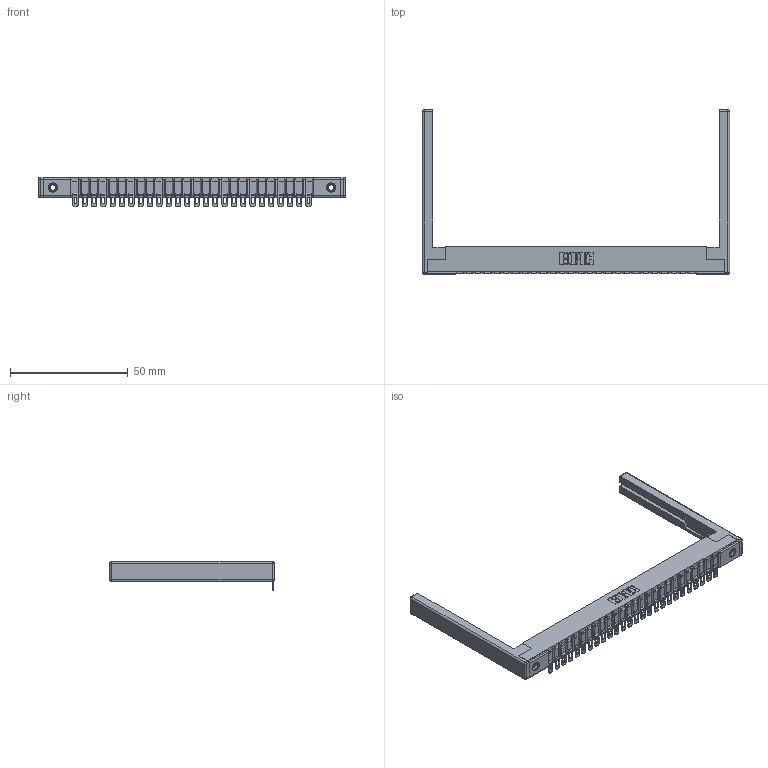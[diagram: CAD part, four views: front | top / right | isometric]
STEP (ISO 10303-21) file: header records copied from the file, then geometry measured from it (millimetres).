
FILE_DESCRIPTION (( 'STEP AP203' ), '1' );
FILE_NAME ('307-026-554-168.STEP', '2019-09-05T02:14:57', ( '' ), ( '' ), 'SwSTEP 2.0', 'SolidWorks 2016', '' );
FILE_SCHEMA (( 'CONFIG_CONTROL_DESIGN' ));
Length unit declared in the file: inch
Products named in the file (5): 307-026-554-168; 307 Part_.156 Dia Mounting Holes; 307-220-068; 345-250-001_345-250-001-102; 307-290-002_554
Assembly tree (31 placements, depth 2):
  307-026-554-168
    307 Part_.156 Dia Mounting Holes
    307-290-002_554  x26
    307-220-068  x2
    345-250-001_345-250-001-102  x2
Bounding box: 130.45 x 69.98 x 12.52 mm (x, y, z)
Volume: 13182.6 mm3; surface area: 20035.2 mm2
Topology: 31 solids, 31 shells, 2405 faces, 7291 edges, 4766 vertices
Faces by surface type: plane 1354, cylinder 973, sphere 62, cone 12, torus 4
Entity records: 27986 total; most frequent: CARTESIAN_POINT 4683, ORIENTED_EDGE 4662, DIRECTION 4581, EDGE_CURVE 2331, VECTOR 1769, LINE 1769, VERTEX_POINT 1508, AXIS2_PLACEMENT_3D 1406
